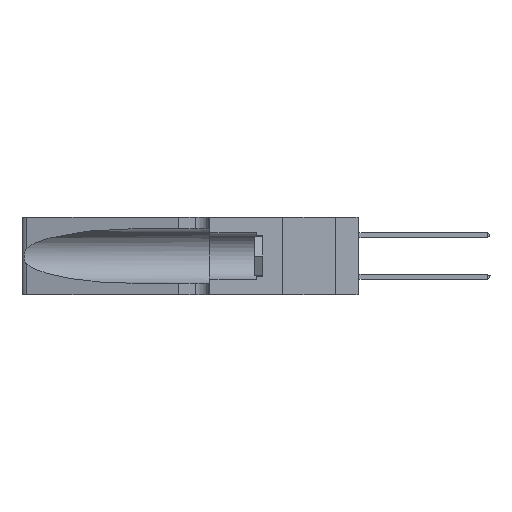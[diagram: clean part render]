
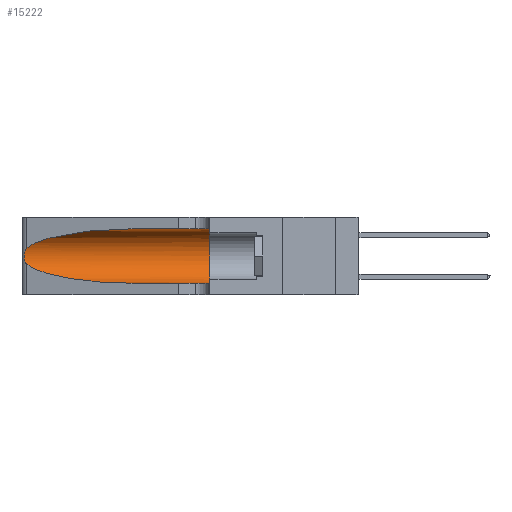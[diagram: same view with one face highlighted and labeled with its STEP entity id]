
A CAD part, left-side view. The second image highlights one B-rep face of the part: STEP entity #15222.
In plain terms, the highlighted cylindrical face has radius 3.308 mm (diameter 6.617 mm), a partial arc.
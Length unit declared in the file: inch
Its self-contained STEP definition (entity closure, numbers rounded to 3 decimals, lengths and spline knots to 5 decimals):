
#459 = CARTESIAN_POINT ( 'NONE',  ( 0.18966, 0.96281, 0.31525 ) ) ;
#1847 = CARTESIAN_POINT ( 'NONE',  ( 0.1305, 0.72297, 0.05475 ) ) ;
#1977 = CARTESIAN_POINT ( 'NONE',  ( 0.1305, 1.61858, 0.31525 ) ) ;
#2309 = CARTESIAN_POINT ( 'NONE',  ( 0.26075, 1.23896, 0.19203 ) ) ;
#3279 = ORIENTED_EDGE ( 'NONE', *, *, #7234, .F. ) ;
#3717 = VECTOR ( 'NONE', #10112, 39.37008 ) ;
#3964 = CARTESIAN_POINT ( 'NONE',  ( 0.1305, 0.72297, 0.31525 ) ) ;
#4488 = ORIENTED_EDGE ( 'NONE', *, *, #5188, .F. ) ;
#5188 = EDGE_CURVE ( 'NONE', #19169, #6812, #29003, .T. ) ;
#5741 = EDGE_LOOP ( 'NONE', ( #18294, #21275, #31440, #16475, #3279, #4488 ) ) ;
#5885 = CIRCLE ( 'NONE', #18659, 0.13025 ) ;
#6812 = VERTEX_POINT ( 'NONE', #11432 ) ;
#6992 = B_SPLINE_CURVE_WITH_KNOTS ( 'NONE', 3,
 ( #24603, #29828, #17213, #29933, #19751, #32454, #2309, #22303, #7160, #15063, #22005, #10360, #23398, #18693 ),
 .UNSPECIFIED., .F., .F.,
 ( 4, 2, 2, 2, 2, 2, 4 ),
 ( 0., 0.00027, 0.00053, 0.00107, 0.0016, 0.00187, 0.00214 ),
 .UNSPECIFIED. ) ;
#7114 = DIRECTION ( 'NONE',  ( 0., 1., 0. ) ) ;
#7160 = CARTESIAN_POINT ( 'NONE',  ( 0.26017, 1.23833, 0.17102 ) ) ;
#7234 = EDGE_CURVE ( 'NONE', #6812, #22675, #5885, .T. ) ;
#7609 = DIRECTION ( 'NONE',  ( 0., -1., 0. ) ) ;
#7945 =( BOUNDED_CURVE ( )  B_SPLINE_CURVE ( 3, ( #24563, #24345, #9114, #1847 ),
 .UNSPECIFIED., .F., .F. ) 
 B_SPLINE_CURVE_WITH_KNOTS ( ( 4, 4 ),
 ( 3.44316, 4.71239 ),
 .UNSPECIFIED. ) 
 CURVE ( )  GEOMETRIC_REPRESENTATION_ITEM ( )  RATIONAL_B_SPLINE_CURVE ( ( 1., 0.87, 0.87, 1. ) ) 
 REPRESENTATION_ITEM ( '' )  );
#9114 = CARTESIAN_POINT ( 'NONE',  ( 0.18966, 0.96281, 0.05475 ) ) ;
#10112 = DIRECTION ( 'NONE',  ( 0., -1., 0. ) ) ;
#10360 = CARTESIAN_POINT ( 'NONE',  ( 0.25639, 1.23186, 0.15144 ) ) ;
#10642 = DIRECTION ( 'NONE',  ( 0., -1., 0. ) ) ;
#10707 = EDGE_CURVE ( 'NONE', #20005, #21469, #6992, .T. ) ;
#11136 = CARTESIAN_POINT ( 'NONE',  ( 0.1305, 0.72297, 0.31525 ) ) ;
#11319 = DIRECTION ( 'NONE',  ( 0., 0., -1. ) ) ;
#11432 = CARTESIAN_POINT ( 'NONE',  ( 0.1305, 0.35, 0.31525 ) ) ;
#11846 = CARTESIAN_POINT ( 'NONE',  ( 0.2373, 1.15595, 0.28018 ) ) ;
#12647 = EDGE_CURVE ( 'NONE', #29926, #22675, #25757, .T. ) ;
#13731 = CARTESIAN_POINT ( 'NONE',  ( 0.25487, 1.22718, 0.14631 ) ) ;
#13908 = VECTOR ( 'NONE', #7609, 39.37008 ) ;
#14236 =( BOUNDED_CURVE ( )  B_SPLINE_CURVE ( 3, ( #3964, #459, #11846, #22328 ),
 .UNSPECIFIED., .F., .F. ) 
 B_SPLINE_CURVE_WITH_KNOTS ( ( 4, 4 ),
 ( 1.5708, 2.84003 ),
 .UNSPECIFIED. ) 
 CURVE ( )  GEOMETRIC_REPRESENTATION_ITEM ( )  RATIONAL_B_SPLINE_CURVE ( ( 1., 0.87, 0.87, 1. ) ) 
 REPRESENTATION_ITEM ( '' )  );
#14602 = CARTESIAN_POINT ( 'NONE',  ( 0.25487, 1.22718, 0.22369 ) ) ;
#15063 = CARTESIAN_POINT ( 'NONE',  ( 0.25856, 1.23593, 0.16098 ) ) ;
#15222 = ADVANCED_FACE ( 'NONE', ( #28344 ), #19286, .F. ) ;
#15351 = EDGE_CURVE ( 'NONE', #19169, #20005, #14236, .T. ) ;
#16018 = CARTESIAN_POINT ( 'NONE',  ( 0.1305, 1.61858, 0.185 ) ) ;
#16475 = ORIENTED_EDGE ( 'NONE', *, *, #12647, .T. ) ;
#17213 = CARTESIAN_POINT ( 'NONE',  ( 0.25639, 1.23184, 0.21858 ) ) ;
#18294 = ORIENTED_EDGE ( 'NONE', *, *, #15351, .T. ) ;
#18659 = AXIS2_PLACEMENT_3D ( 'NONE', #22245, #7114, #26989 ) ;
#18693 = CARTESIAN_POINT ( 'NONE',  ( 0.25487, 1.22718, 0.14631 ) ) ;
#19169 = VERTEX_POINT ( 'NONE', #11136 ) ;
#19286 = CYLINDRICAL_SURFACE ( 'NONE', #19911, 0.13025 ) ;
#19751 = CARTESIAN_POINT ( 'NONE',  ( 0.25854, 1.2359, 0.20912 ) ) ;
#19911 = AXIS2_PLACEMENT_3D ( 'NONE', #16018, #10642, #11319 ) ;
#20005 = VERTEX_POINT ( 'NONE', #14602 ) ;
#21275 = ORIENTED_EDGE ( 'NONE', *, *, #10707, .T. ) ;
#21469 = VERTEX_POINT ( 'NONE', #13731 ) ;
#21752 = CARTESIAN_POINT ( 'NONE',  ( 0.1305, 0.72297, 0.05475 ) ) ;
#22005 = CARTESIAN_POINT ( 'NONE',  ( 0.25789, 1.23486, 0.15765 ) ) ;
#22245 = CARTESIAN_POINT ( 'NONE',  ( 0.1305, 0.35, 0.185 ) ) ;
#22303 = CARTESIAN_POINT ( 'NONE',  ( 0.26075, 1.23896, 0.178 ) ) ;
#22328 = CARTESIAN_POINT ( 'NONE',  ( 0.25487, 1.22718, 0.22369 ) ) ;
#22675 = VERTEX_POINT ( 'NONE', #26625 ) ;
#23398 = CARTESIAN_POINT ( 'NONE',  ( 0.25555, 1.22993, 0.14849 ) ) ;
#24345 = CARTESIAN_POINT ( 'NONE',  ( 0.2373, 1.15595, 0.08982 ) ) ;
#24563 = CARTESIAN_POINT ( 'NONE',  ( 0.25487, 1.22718, 0.14631 ) ) ;
#24603 = CARTESIAN_POINT ( 'NONE',  ( 0.25487, 1.22718, 0.22369 ) ) ;
#25757 = LINE ( 'NONE', #32235, #13908 ) ;
#26625 = CARTESIAN_POINT ( 'NONE',  ( 0.1305, 0.35, 0.05475 ) ) ;
#26989 = DIRECTION ( 'NONE',  ( 0., 0., 1. ) ) ;
#28344 = FACE_OUTER_BOUND ( 'NONE', #5741, .T. ) ;
#29003 = LINE ( 'NONE', #1977, #3717 ) ;
#29828 = CARTESIAN_POINT ( 'NONE',  ( 0.25555, 1.22994, 0.2215 ) ) ;
#29926 = VERTEX_POINT ( 'NONE', #21752 ) ;
#29933 = CARTESIAN_POINT ( 'NONE',  ( 0.25787, 1.23484, 0.2124 ) ) ;
#30508 = EDGE_CURVE ( 'NONE', #21469, #29926, #7945, .T. ) ;
#31440 = ORIENTED_EDGE ( 'NONE', *, *, #30508, .T. ) ;
#32235 = CARTESIAN_POINT ( 'NONE',  ( 0.1305, 1.61858, 0.05475 ) ) ;
#32454 = CARTESIAN_POINT ( 'NONE',  ( 0.26018, 1.23835, 0.19895 ) ) ;
